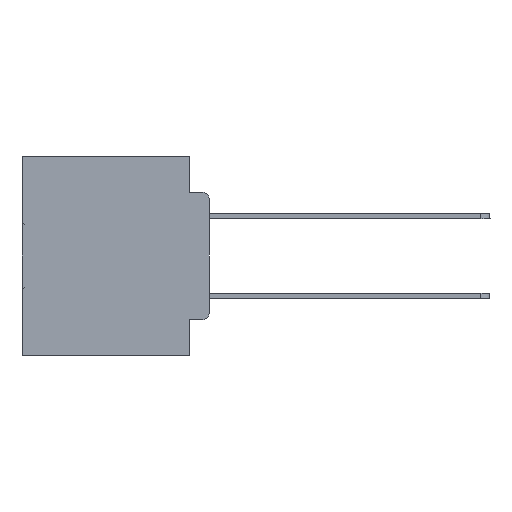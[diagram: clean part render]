
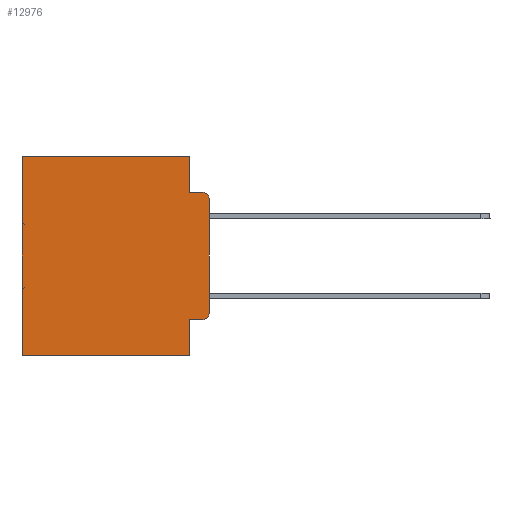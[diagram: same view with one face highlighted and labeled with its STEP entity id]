
A CAD part, left-side view. The second image highlights one B-rep face of the part: STEP entity #12976.
In plain terms, the highlighted planar face has unit normal (-1, 0, 0).
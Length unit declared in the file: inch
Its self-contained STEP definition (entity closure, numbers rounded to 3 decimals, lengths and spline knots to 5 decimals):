
#169 = VERTEX_POINT ( 'NONE', #36126 ) ;
#1559 = ORIENTED_EDGE ( 'NONE', *, *, #12423, .T. ) ;
#1589 = CARTESIAN_POINT ( 'NONE',  ( 0.298, 0.051, 0. ) ) ;
#2103 = CARTESIAN_POINT ( 'NONE',  ( 0.298, 0., 0. ) ) ;
#2552 = VECTOR ( 'NONE', #19998, 39.37008 ) ;
#2987 = DIRECTION ( 'NONE',  ( 0., -1., 0. ) ) ;
#3101 = VECTOR ( 'NONE', #24989, 39.37008 ) ;
#3761 = LINE ( 'NONE', #35086, #33327 ) ;
#4058 = ORIENTED_EDGE ( 'NONE', *, *, #35213, .F. ) ;
#5529 = VERTEX_POINT ( 'NONE', #28730 ) ;
#7141 = ORIENTED_EDGE ( 'NONE', *, *, #26292, .F. ) ;
#7441 = LINE ( 'NONE', #2103, #15951 ) ;
#7683 = EDGE_CURVE ( 'NONE', #5529, #11830, #21545, .T. ) ;
#8144 = DIRECTION ( 'NONE',  ( 0., 0., -1. ) ) ;
#8247 = VERTEX_POINT ( 'NONE', #29831 ) ;
#8351 = EDGE_CURVE ( 'NONE', #33069, #18280, #36669, .T. ) ;
#8790 = CARTESIAN_POINT ( 'NONE',  ( 0.298, 0.051, 0. ) ) ;
#9373 = DIRECTION ( 'NONE',  ( 0., 1., 0. ) ) ;
#9608 = ORIENTED_EDGE ( 'NONE', *, *, #12312, .T. ) ;
#9648 = CARTESIAN_POINT ( 'NONE',  ( 0.298, 0.051, 0. ) ) ;
#9945 = DIRECTION ( 'NONE',  ( 0., 1., 0. ) ) ;
#10777 = CARTESIAN_POINT ( 'NONE',  ( 0.298, 0.051, -0.4115 ) ) ;
#10900 = DIRECTION ( 'NONE',  ( 0., -1., 0. ) ) ;
#11692 = CARTESIAN_POINT ( 'NONE',  ( 0.298, 0.051, -0.0885 ) ) ;
#11792 = AXIS2_PLACEMENT_3D ( 'NONE', #16313, #19322, #33926 ) ;
#11830 = VERTEX_POINT ( 'NONE', #35346 ) ;
#12234 = ORIENTED_EDGE ( 'NONE', *, *, #8351, .F. ) ;
#12312 = EDGE_CURVE ( 'NONE', #28398, #16344, #18096, .T. ) ;
#12333 = LINE ( 'NONE', #8790, #2552 ) ;
#12423 = EDGE_CURVE ( 'NONE', #33069, #5529, #3761, .T. ) ;
#12847 = CARTESIAN_POINT ( 'NONE',  ( 0.298, 0.02, -0.0885 ) ) ;
#12976 = ADVANCED_FACE ( 'NONE', ( #25704 ), #22548, .F. ) ;
#13223 = ORIENTED_EDGE ( 'NONE', *, *, #19650, .T. ) ;
#13720 = VERTEX_POINT ( 'NONE', #12847 ) ;
#15666 = EDGE_CURVE ( 'NONE', #8247, #11830, #23262, .T. ) ;
#15951 = VECTOR ( 'NONE', #8144, 39.37008 ) ;
#16141 = VECTOR ( 'NONE', #26144, 39.37008 ) ;
#16313 = CARTESIAN_POINT ( 'NONE',  ( 0.298, 0.02, -0.1085 ) ) ;
#16315 = EDGE_LOOP ( 'NONE', ( #35855, #17606, #7141, #12234, #1559, #31889, #22441, #4058, #9608, #13223 ) ) ;
#16331 = CARTESIAN_POINT ( 'NONE',  ( 0.298, 0., -0.3915 ) ) ;
#16344 = VERTEX_POINT ( 'NONE', #17884 ) ;
#16509 = DIRECTION ( 'NONE',  ( 0., 0., -1. ) ) ;
#17039 = AXIS2_PLACEMENT_3D ( 'NONE', #31177, #36891, #16509 ) ;
#17606 = ORIENTED_EDGE ( 'NONE', *, *, #27224, .T. ) ;
#17788 = CARTESIAN_POINT ( 'NONE',  ( 0.298, 0., -0.5 ) ) ;
#17884 = CARTESIAN_POINT ( 'NONE',  ( 0.298, 0.02, -0.4115 ) ) ;
#18096 = LINE ( 'NONE', #28094, #26628 ) ;
#18280 = VERTEX_POINT ( 'NONE', #22664 ) ;
#19260 = VECTOR ( 'NONE', #9373, 39.37008 ) ;
#19322 = DIRECTION ( 'NONE',  ( -1., 0., 0. ) ) ;
#19650 = EDGE_CURVE ( 'NONE', #16344, #22300, #21939, .T. ) ;
#19998 = DIRECTION ( 'NONE',  ( 0., 0., -1. ) ) ;
#21545 = LINE ( 'NONE', #23244, #16141 ) ;
#21939 = CIRCLE ( 'NONE', #27751, 0.02 ) ;
#22178 = LINE ( 'NONE', #11692, #33762 ) ;
#22300 = VERTEX_POINT ( 'NONE', #16331 ) ;
#22441 = ORIENTED_EDGE ( 'NONE', *, *, #15666, .F. ) ;
#22548 = PLANE ( 'NONE',  #17039 ) ;
#22664 = CARTESIAN_POINT ( 'NONE',  ( 0.298, 0.051, -0.0885 ) ) ;
#23244 = CARTESIAN_POINT ( 'NONE',  ( 0.298, 0.473, 0. ) ) ;
#23262 = LINE ( 'NONE', #17788, #19260 ) ;
#24989 = DIRECTION ( 'NONE',  ( 0., 0., -1. ) ) ;
#25297 = EDGE_CURVE ( 'NONE', #169, #22300, #7441, .T. ) ;
#25704 = FACE_OUTER_BOUND ( 'NONE', #16315, .T. ) ;
#26144 = DIRECTION ( 'NONE',  ( 0., 0., -1. ) ) ;
#26292 = EDGE_CURVE ( 'NONE', #18280, #13720, #22178, .T. ) ;
#26628 = VECTOR ( 'NONE', #10900, 39.37008 ) ;
#27224 = EDGE_CURVE ( 'NONE', #169, #13720, #33687, .T. ) ;
#27751 = AXIS2_PLACEMENT_3D ( 'NONE', #36106, #27887, #33337 ) ;
#27887 = DIRECTION ( 'NONE',  ( -1., 0., 0. ) ) ;
#28094 = CARTESIAN_POINT ( 'NONE',  ( 0.298, 0.051, -0.4115 ) ) ;
#28398 = VERTEX_POINT ( 'NONE', #10777 ) ;
#28730 = CARTESIAN_POINT ( 'NONE',  ( 0.298, 0.473, 0. ) ) ;
#29831 = CARTESIAN_POINT ( 'NONE',  ( 0.298, 0.051, -0.5 ) ) ;
#31177 = CARTESIAN_POINT ( 'NONE',  ( 0.298, 0., 0. ) ) ;
#31889 = ORIENTED_EDGE ( 'NONE', *, *, #7683, .T. ) ;
#33069 = VERTEX_POINT ( 'NONE', #1589 ) ;
#33327 = VECTOR ( 'NONE', #9945, 39.37008 ) ;
#33337 = DIRECTION ( 'NONE',  ( 0., 0., -1. ) ) ;
#33687 = CIRCLE ( 'NONE', #11792, 0.02 ) ;
#33762 = VECTOR ( 'NONE', #2987, 39.37008 ) ;
#33926 = DIRECTION ( 'NONE',  ( 0., 0., -1. ) ) ;
#35086 = CARTESIAN_POINT ( 'NONE',  ( 0.298, 0., 0. ) ) ;
#35213 = EDGE_CURVE ( 'NONE', #28398, #8247, #12333, .T. ) ;
#35346 = CARTESIAN_POINT ( 'NONE',  ( 0.298, 0.473, -0.5 ) ) ;
#35855 = ORIENTED_EDGE ( 'NONE', *, *, #25297, .F. ) ;
#36106 = CARTESIAN_POINT ( 'NONE',  ( 0.298, 0.02, -0.3915 ) ) ;
#36126 = CARTESIAN_POINT ( 'NONE',  ( 0.298, 0., -0.1085 ) ) ;
#36669 = LINE ( 'NONE', #9648, #3101 ) ;
#36891 = DIRECTION ( 'NONE',  ( 1., 0., 0. ) ) ;
